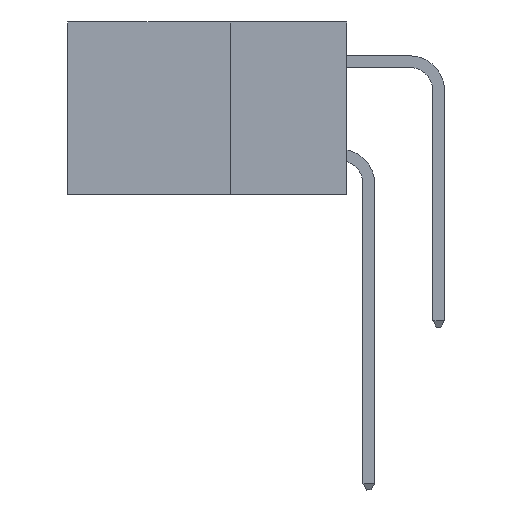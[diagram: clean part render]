
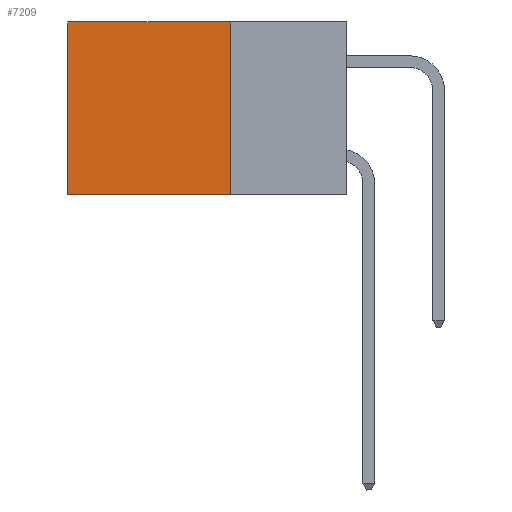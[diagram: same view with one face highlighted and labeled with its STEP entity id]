
A CAD part, left-side view. The second image highlights one B-rep face of the part: STEP entity #7209.
In plain terms, the highlighted planar face has unit normal (-1, 0, 0).
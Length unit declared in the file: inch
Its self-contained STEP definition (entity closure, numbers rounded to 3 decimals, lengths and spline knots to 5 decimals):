
#386 = EDGE_CURVE ( 'NONE', #31273, #19632, #13044, .T. ) ;
#420 = EDGE_CURVE ( 'NONE', #15943, #12616, #27314, .T. ) ;
#1287 = FACE_OUTER_BOUND ( 'NONE', #18554, .T. ) ;
#1957 = PLANE ( 'NONE',  #23607 ) ;
#2414 = DIRECTION ( 'NONE',  ( 0., 1., 0. ) ) ;
#3448 = LINE ( 'NONE', #21400, #3745 ) ;
#3618 = CARTESIAN_POINT ( 'NONE',  ( 0.2875, 0.25, 0. ) ) ;
#3745 = VECTOR ( 'NONE', #18777, 39.37008 ) ;
#3926 = VECTOR ( 'NONE', #2414, 39.37008 ) ;
#4064 = DIRECTION ( 'NONE',  ( 0., 0., -1. ) ) ;
#5732 = ORIENTED_EDGE ( 'NONE', *, *, #420, .T. ) ;
#7209 = ADVANCED_FACE ( 'NONE', ( #1287 ), #1957, .F. ) ;
#9006 = CARTESIAN_POINT ( 'NONE',  ( 0.2875, 0.6, -0.37 ) ) ;
#12616 = VERTEX_POINT ( 'NONE', #24434 ) ;
#12937 = CARTESIAN_POINT ( 'NONE',  ( 0.2875, 0.6, 0. ) ) ;
#13044 = LINE ( 'NONE', #16006, #3926 ) ;
#14703 = DIRECTION ( 'NONE',  ( 1., 0., 0. ) ) ;
#15906 = DIRECTION ( 'NONE',  ( 0., 0., -1. ) ) ;
#15943 = VERTEX_POINT ( 'NONE', #31123 ) ;
#16006 = CARTESIAN_POINT ( 'NONE',  ( 0.2875, 0.25, -0.37 ) ) ;
#17067 = VECTOR ( 'NONE', #15906, 39.37008 ) ;
#18554 = EDGE_LOOP ( 'NONE', ( #33165, #30224, #27651, #5732 ) ) ;
#18777 = DIRECTION ( 'NONE',  ( 0., 0., -1. ) ) ;
#19632 = VERTEX_POINT ( 'NONE', #9006 ) ;
#21400 = CARTESIAN_POINT ( 'NONE',  ( 0.2875, 0.25, 0. ) ) ;
#23607 = AXIS2_PLACEMENT_3D ( 'NONE', #33496, #14703, #4064 ) ;
#24434 = CARTESIAN_POINT ( 'NONE',  ( 0.2875, 0.6, 0. ) ) ;
#26158 = VECTOR ( 'NONE', #32882, 39.37008 ) ;
#26331 = LINE ( 'NONE', #12937, #17067 ) ;
#27314 = LINE ( 'NONE', #3618, #26158 ) ;
#27651 = ORIENTED_EDGE ( 'NONE', *, *, #33161, .F. ) ;
#29087 = CARTESIAN_POINT ( 'NONE',  ( 0.2875, 0.25, -0.37 ) ) ;
#30224 = ORIENTED_EDGE ( 'NONE', *, *, #386, .F. ) ;
#30892 = EDGE_CURVE ( 'NONE', #12616, #19632, #26331, .T. ) ;
#31123 = CARTESIAN_POINT ( 'NONE',  ( 0.2875, 0.25, 0. ) ) ;
#31273 = VERTEX_POINT ( 'NONE', #29087 ) ;
#32882 = DIRECTION ( 'NONE',  ( 0., 1., 0. ) ) ;
#33161 = EDGE_CURVE ( 'NONE', #15943, #31273, #3448, .T. ) ;
#33165 = ORIENTED_EDGE ( 'NONE', *, *, #30892, .T. ) ;
#33496 = CARTESIAN_POINT ( 'NONE',  ( 0.2875, 0.25, 0. ) ) ;
